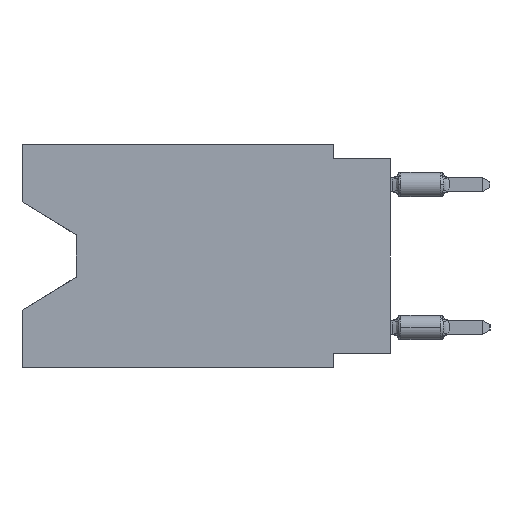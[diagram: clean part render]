
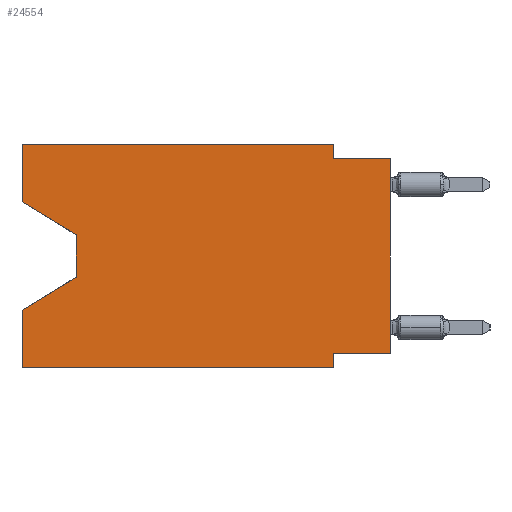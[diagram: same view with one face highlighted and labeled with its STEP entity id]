
A CAD part, left-side view. The second image highlights one B-rep face of the part: STEP entity #24554.
In plain terms, the highlighted planar face has unit normal (-1, 0, 0).
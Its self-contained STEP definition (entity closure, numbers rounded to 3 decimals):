
#30 = EDGE_CURVE ( 'NONE', #13302, #28627, #7342, .T. ) ;
#56 = CARTESIAN_POINT ( 'NONE',  ( 0., 16.383, 0. ) ) ;
#278 = VERTEX_POINT ( 'NONE', #14650 ) ;
#351 = VERTEX_POINT ( 'NONE', #27900 ) ;
#462 = CARTESIAN_POINT ( 'NONE',  ( 0., 0., -0.635 ) ) ;
#1241 = EDGE_CURVE ( 'NONE', #7985, #11278, #24997, .T. ) ;
#2402 = PLANE ( 'NONE',  #12220 ) ;
#2972 = ORIENTED_EDGE ( 'NONE', *, *, #26079, .T. ) ;
#4921 = FACE_OUTER_BOUND ( 'NONE', #29458, .T. ) ;
#5848 = DIRECTION ( 'NONE',  ( 0., -1., 0. ) ) ;
#6004 = DIRECTION ( 'NONE',  ( 0., 0., 1. ) ) ;
#6301 = VECTOR ( 'NONE', #5848, 1000. ) ;
#6512 = VERTEX_POINT ( 'NONE', #18206 ) ;
#6893 = ORIENTED_EDGE ( 'NONE', *, *, #19761, .F. ) ;
#7311 = DIRECTION ( 'NONE',  ( 0., 0., 1. ) ) ;
#7342 = LINE ( 'NONE', #17728, #25499 ) ;
#7352 = LINE ( 'NONE', #29364, #33579 ) ;
#7777 = DIRECTION ( 'NONE',  ( 0., -1., 0. ) ) ;
#7985 = VERTEX_POINT ( 'NONE', #20226 ) ;
#9078 = LINE ( 'NONE', #21987, #6301 ) ;
#9188 = ORIENTED_EDGE ( 'NONE', *, *, #10778, .T. ) ;
#9250 = VECTOR ( 'NONE', #18351, 1000. ) ;
#9342 = VECTOR ( 'NONE', #14992, 1000. ) ;
#9370 = EDGE_CURVE ( 'NONE', #11278, #278, #9078, .T. ) ;
#9614 = CARTESIAN_POINT ( 'NONE',  ( 0., 16.383, 0. ) ) ;
#9854 = ORIENTED_EDGE ( 'NONE', *, *, #15500, .T. ) ;
#10001 = ORIENTED_EDGE ( 'NONE', *, *, #1241, .F. ) ;
#10698 = CARTESIAN_POINT ( 'NONE',  ( 0., 2.54, -0.635 ) ) ;
#10778 = EDGE_CURVE ( 'NONE', #16557, #28627, #23549, .T. ) ;
#10998 = VECTOR ( 'NONE', #16724, 1000. ) ;
#11278 = VERTEX_POINT ( 'NONE', #16151 ) ;
#12076 = CARTESIAN_POINT ( 'NONE',  ( 0., 16.383, -9.906 ) ) ;
#12220 = AXIS2_PLACEMENT_3D ( 'NONE', #56, #21906, #18529 ) ;
#12436 = VECTOR ( 'NONE', #7777, 1000. ) ;
#12496 = CARTESIAN_POINT ( 'NONE',  ( 0., 0., 0. ) ) ;
#12714 = ORIENTED_EDGE ( 'NONE', *, *, #30, .F. ) ;
#12846 = VECTOR ( 'NONE', #30726, 1000. ) ;
#12959 = EDGE_CURVE ( 'NONE', #26874, #13302, #7352, .T. ) ;
#13302 = VERTEX_POINT ( 'NONE', #20567 ) ;
#14122 = ORIENTED_EDGE ( 'NONE', *, *, #12959, .F. ) ;
#14567 = VECTOR ( 'NONE', #7311, 1000. ) ;
#14650 = CARTESIAN_POINT ( 'NONE',  ( 0., 2.54, 0. ) ) ;
#14992 = DIRECTION ( 'NONE',  ( 0., 0., 1. ) ) ;
#15370 = ORIENTED_EDGE ( 'NONE', *, *, #24489, .F. ) ;
#15500 = EDGE_CURVE ( 'NONE', #7985, #351, #31127, .T. ) ;
#15718 = ORIENTED_EDGE ( 'NONE', *, *, #16712, .T. ) ;
#16151 = CARTESIAN_POINT ( 'NONE',  ( 0., 16.383, 0. ) ) ;
#16557 = VERTEX_POINT ( 'NONE', #17167 ) ;
#16712 = EDGE_CURVE ( 'NONE', #26874, #33645, #31836, .T. ) ;
#16724 = DIRECTION ( 'NONE',  ( 0., 0., -1. ) ) ;
#16869 = VERTEX_POINT ( 'NONE', #10698 ) ;
#17167 = CARTESIAN_POINT ( 'NONE',  ( 0., 16.383, -9.906 ) ) ;
#17228 = DIRECTION ( 'NONE',  ( 0., 0., -1. ) ) ;
#17286 = LINE ( 'NONE', #33403, #12846 ) ;
#17728 = CARTESIAN_POINT ( 'NONE',  ( 0., 2.54, -9.906 ) ) ;
#18206 = CARTESIAN_POINT ( 'NONE',  ( 0., 16.383, -7.36 ) ) ;
#18351 = DIRECTION ( 'NONE',  ( 0., -1., 0. ) ) ;
#18529 = DIRECTION ( 'NONE',  ( 0., 0., -1. ) ) ;
#19753 = VECTOR ( 'NONE', #6004, 1000. ) ;
#19761 = EDGE_CURVE ( 'NONE', #278, #16869, #19932, .T. ) ;
#19932 = LINE ( 'NONE', #30833, #23884 ) ;
#20226 = CARTESIAN_POINT ( 'NONE',  ( 0., 16.383, -2.546 ) ) ;
#20567 = CARTESIAN_POINT ( 'NONE',  ( 0., 2.54, -9.271 ) ) ;
#20739 = CARTESIAN_POINT ( 'NONE',  ( 0., 16.383, -2.546 ) ) ;
#20880 = LINE ( 'NONE', #24094, #10998 ) ;
#20950 = CARTESIAN_POINT ( 'NONE',  ( 0., 0., -9.271 ) ) ;
#21033 = CARTESIAN_POINT ( 'NONE',  ( 0., 0., -0.635 ) ) ;
#21330 = ORIENTED_EDGE ( 'NONE', *, *, #23258, .F. ) ;
#21382 = LINE ( 'NONE', #21033, #12436 ) ;
#21906 = DIRECTION ( 'NONE',  ( 1., 0., 0. ) ) ;
#21987 = CARTESIAN_POINT ( 'NONE',  ( 0., 16.383, 0. ) ) ;
#22623 = ORIENTED_EDGE ( 'NONE', *, *, #9370, .F. ) ;
#23258 = EDGE_CURVE ( 'NONE', #16869, #33645, #21382, .T. ) ;
#23549 = LINE ( 'NONE', #12076, #9250 ) ;
#23641 = DIRECTION ( 'NONE',  ( 0., 0., -1. ) ) ;
#23884 = VECTOR ( 'NONE', #17228, 1000. ) ;
#24094 = CARTESIAN_POINT ( 'NONE',  ( 0., 13.97, -4.013 ) ) ;
#24489 = EDGE_CURVE ( 'NONE', #16557, #6512, #30933, .T. ) ;
#24554 = ADVANCED_FACE ( 'NONE', ( #4921 ), #2402, .F. ) ;
#24997 = LINE ( 'NONE', #35386, #19753 ) ;
#25499 = VECTOR ( 'NONE', #23641, 1000. ) ;
#25925 = CARTESIAN_POINT ( 'NONE',  ( 0., 2.54, -9.906 ) ) ;
#26079 = EDGE_CURVE ( 'NONE', #35322, #6512, #17286, .T. ) ;
#26874 = VERTEX_POINT ( 'NONE', #20950 ) ;
#27030 = DIRECTION ( 'NONE',  ( 0., 1., 0. ) ) ;
#27431 = CARTESIAN_POINT ( 'NONE',  ( 0., 13.97, -5.893 ) ) ;
#27900 = CARTESIAN_POINT ( 'NONE',  ( 0., 13.97, -4.013 ) ) ;
#27962 = VECTOR ( 'NONE', #34176, 1000. ) ;
#28627 = VERTEX_POINT ( 'NONE', #25925 ) ;
#29364 = CARTESIAN_POINT ( 'NONE',  ( 0., 0., -9.271 ) ) ;
#29458 = EDGE_LOOP ( 'NONE', ( #9854, #33509, #2972, #15370, #9188, #12714, #14122, #15718, #21330, #6893, #22623, #10001 ) ) ;
#30726 = DIRECTION ( 'NONE',  ( 0., 0.855, -0.519 ) ) ;
#30833 = CARTESIAN_POINT ( 'NONE',  ( 0., 2.54, 0. ) ) ;
#30933 = LINE ( 'NONE', #9614, #9342 ) ;
#31127 = LINE ( 'NONE', #20739, #27962 ) ;
#31836 = LINE ( 'NONE', #12496, #14567 ) ;
#33403 = CARTESIAN_POINT ( 'NONE',  ( 0., 13.97, -5.893 ) ) ;
#33509 = ORIENTED_EDGE ( 'NONE', *, *, #34858, .T. ) ;
#33579 = VECTOR ( 'NONE', #27030, 1000. ) ;
#33645 = VERTEX_POINT ( 'NONE', #462 ) ;
#34176 = DIRECTION ( 'NONE',  ( 0., -0.855, -0.519 ) ) ;
#34858 = EDGE_CURVE ( 'NONE', #351, #35322, #20880, .T. ) ;
#35322 = VERTEX_POINT ( 'NONE', #27431 ) ;
#35386 = CARTESIAN_POINT ( 'NONE',  ( 0., 16.383, 0. ) ) ;
